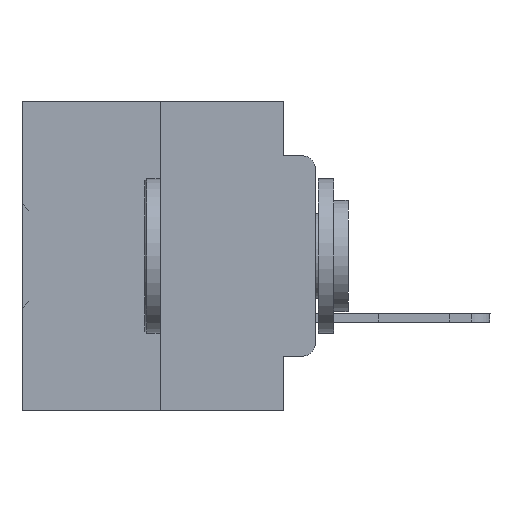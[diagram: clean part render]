
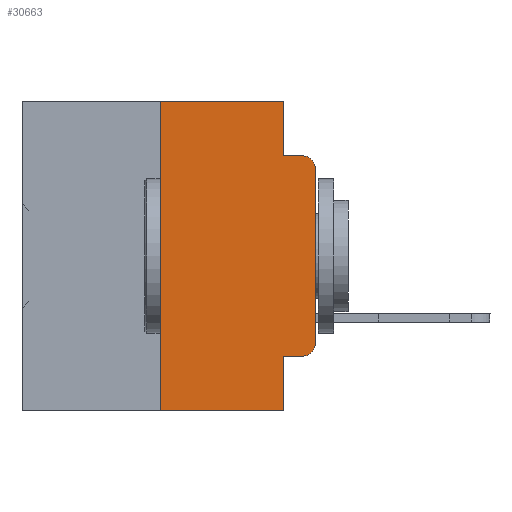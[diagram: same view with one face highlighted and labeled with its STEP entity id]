
A CAD part, left-side view. The second image highlights one B-rep face of the part: STEP entity #30663.
In plain terms, the highlighted planar face has unit normal (-1, 0, 0).
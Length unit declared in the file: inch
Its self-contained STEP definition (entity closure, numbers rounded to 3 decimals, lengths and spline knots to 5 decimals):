
#653 = EDGE_CURVE ( 'NONE', #27274, #29339, #15769, .T. ) ;
#1051 = AXIS2_PLACEMENT_3D ( 'NONE', #27314, #12923, #24215 ) ;
#1223 = CARTESIAN_POINT ( 'NONE',  ( 0., 0.25, 0. ) ) ;
#2347 = ORIENTED_EDGE ( 'NONE', *, *, #5099, .F. ) ;
#2530 = VECTOR ( 'NONE', #38214, 39.37008 ) ;
#3540 = EDGE_CURVE ( 'NONE', #31418, #37774, #5911, .T. ) ;
#4879 = DIRECTION ( 'NONE',  ( 0., 0., 1. ) ) ;
#5099 = EDGE_CURVE ( 'NONE', #31418, #29339, #5110, .T. ) ;
#5110 = LINE ( 'NONE', #19551, #16150 ) ;
#5453 = CARTESIAN_POINT ( 'NONE',  ( 0., 0.051, 0. ) ) ;
#5911 = LINE ( 'NONE', #11394, #26783 ) ;
#6573 = CARTESIAN_POINT ( 'NONE',  ( 0., 0.25, -0.5 ) ) ;
#6642 = DIRECTION ( 'NONE',  ( 0., 0., -1. ) ) ;
#7090 = LINE ( 'NONE', #1223, #31521 ) ;
#7589 = ORIENTED_EDGE ( 'NONE', *, *, #15811, .T. ) ;
#7619 = DIRECTION ( 'NONE',  ( 0., -1., 0. ) ) ;
#9211 = VERTEX_POINT ( 'NONE', #33535 ) ;
#9321 = DIRECTION ( 'NONE',  ( 0., 0., -1. ) ) ;
#11331 = CARTESIAN_POINT ( 'NONE',  ( 0., 0.02, -0.3915 ) ) ;
#11394 = CARTESIAN_POINT ( 'NONE',  ( 0., 0.051, -0.4115 ) ) ;
#12128 = DIRECTION ( 'NONE',  ( 1., 0., 0. ) ) ;
#12611 = ORIENTED_EDGE ( 'NONE', *, *, #26985, .F. ) ;
#12923 = DIRECTION ( 'NONE',  ( -1., 0., 0. ) ) ;
#13145 = DIRECTION ( 'NONE',  ( 0., 0., 1. ) ) ;
#13280 = EDGE_LOOP ( 'NONE', ( #17221, #7589, #32974, #35459, #12611, #26926, #21923, #2347, #28087, #18136 ) ) ;
#13389 = VECTOR ( 'NONE', #28223, 39.37008 ) ;
#13776 = CIRCLE ( 'NONE', #26202, 0.02 ) ;
#13886 = VERTEX_POINT ( 'NONE', #20137 ) ;
#13948 = VERTEX_POINT ( 'NONE', #20501 ) ;
#15060 = PLANE ( 'NONE',  #24392 ) ;
#15769 = LINE ( 'NONE', #36576, #2530 ) ;
#15795 = CARTESIAN_POINT ( 'NONE',  ( 0., 0.02, -0.4115 ) ) ;
#15811 = EDGE_CURVE ( 'NONE', #13886, #13948, #17973, .T. ) ;
#16150 = VECTOR ( 'NONE', #17020, 39.37008 ) ;
#17020 = DIRECTION ( 'NONE',  ( 0., 0., -1. ) ) ;
#17221 = ORIENTED_EDGE ( 'NONE', *, *, #30911, .T. ) ;
#17737 = VECTOR ( 'NONE', #7619, 39.37008 ) ;
#17853 = VERTEX_POINT ( 'NONE', #26284 ) ;
#17931 = LINE ( 'NONE', #5453, #35077 ) ;
#17973 = CIRCLE ( 'NONE', #1051, 0.02 ) ;
#18136 = ORIENTED_EDGE ( 'NONE', *, *, #21850, .T. ) ;
#18350 = CARTESIAN_POINT ( 'NONE',  ( 0., 0.473, 0. ) ) ;
#19011 = CARTESIAN_POINT ( 'NONE',  ( 0., 0.25, 0. ) ) ;
#19551 = CARTESIAN_POINT ( 'NONE',  ( 0., 0.051, 0. ) ) ;
#20137 = CARTESIAN_POINT ( 'NONE',  ( 0., 0., -0.1085 ) ) ;
#20501 = CARTESIAN_POINT ( 'NONE',  ( 0., 0.02, -0.0885 ) ) ;
#21272 = FACE_OUTER_BOUND ( 'NONE', #13280, .T. ) ;
#21850 = EDGE_CURVE ( 'NONE', #37774, #17853, #13776, .T. ) ;
#21923 = ORIENTED_EDGE ( 'NONE', *, *, #653, .T. ) ;
#22612 = LINE ( 'NONE', #34507, #35569 ) ;
#22829 = LINE ( 'NONE', #23209, #17737 ) ;
#23209 = CARTESIAN_POINT ( 'NONE',  ( 0., 0.051, -0.0885 ) ) ;
#23402 = DIRECTION ( 'NONE',  ( -1., 0., 0. ) ) ;
#23604 = CARTESIAN_POINT ( 'NONE',  ( 0., 0.051, -0.5 ) ) ;
#24215 = DIRECTION ( 'NONE',  ( 0., 0., -1. ) ) ;
#24392 = AXIS2_PLACEMENT_3D ( 'NONE', #18350, #12128, #6642 ) ;
#25231 = EDGE_CURVE ( 'NONE', #9211, #13948, #22829, .T. ) ;
#26202 = AXIS2_PLACEMENT_3D ( 'NONE', #11331, #23402, #38192 ) ;
#26284 = CARTESIAN_POINT ( 'NONE',  ( 0., 0., -0.3915 ) ) ;
#26783 = VECTOR ( 'NONE', #29687, 39.37008 ) ;
#26926 = ORIENTED_EDGE ( 'NONE', *, *, #36924, .F. ) ;
#26985 = EDGE_CURVE ( 'NONE', #27307, #32559, #35047, .T. ) ;
#27274 = VERTEX_POINT ( 'NONE', #6573 ) ;
#27307 = VERTEX_POINT ( 'NONE', #19011 ) ;
#27314 = CARTESIAN_POINT ( 'NONE',  ( 0., 0.02, -0.1085 ) ) ;
#28087 = ORIENTED_EDGE ( 'NONE', *, *, #3540, .T. ) ;
#28223 = DIRECTION ( 'NONE',  ( 0., -1., 0. ) ) ;
#29339 = VERTEX_POINT ( 'NONE', #23604 ) ;
#29687 = DIRECTION ( 'NONE',  ( 0., -1., 0. ) ) ;
#30120 = CARTESIAN_POINT ( 'NONE',  ( 0., 0.051, 0. ) ) ;
#30663 = ADVANCED_FACE ( 'NONE', ( #21272 ), #15060, .F. ) ;
#30911 = EDGE_CURVE ( 'NONE', #17853, #13886, #22612, .T. ) ;
#31278 = CARTESIAN_POINT ( 'NONE',  ( 0., 0.051, -0.4115 ) ) ;
#31418 = VERTEX_POINT ( 'NONE', #31278 ) ;
#31521 = VECTOR ( 'NONE', #13145, 39.37008 ) ;
#32559 = VERTEX_POINT ( 'NONE', #30120 ) ;
#32974 = ORIENTED_EDGE ( 'NONE', *, *, #25231, .F. ) ;
#33535 = CARTESIAN_POINT ( 'NONE',  ( 0., 0.051, -0.0885 ) ) ;
#33855 = EDGE_CURVE ( 'NONE', #32559, #9211, #17931, .T. ) ;
#34507 = CARTESIAN_POINT ( 'NONE',  ( 0., 0., 0. ) ) ;
#35047 = LINE ( 'NONE', #37953, #13389 ) ;
#35077 = VECTOR ( 'NONE', #9321, 39.37008 ) ;
#35459 = ORIENTED_EDGE ( 'NONE', *, *, #33855, .F. ) ;
#35569 = VECTOR ( 'NONE', #4879, 39.37008 ) ;
#36576 = CARTESIAN_POINT ( 'NONE',  ( 0., 0.473, -0.5 ) ) ;
#36924 = EDGE_CURVE ( 'NONE', #27274, #27307, #7090, .T. ) ;
#37774 = VERTEX_POINT ( 'NONE', #15795 ) ;
#37953 = CARTESIAN_POINT ( 'NONE',  ( 0., 0.473, 0. ) ) ;
#38192 = DIRECTION ( 'NONE',  ( 0., 0., -1. ) ) ;
#38214 = DIRECTION ( 'NONE',  ( 0., -1., 0. ) ) ;
